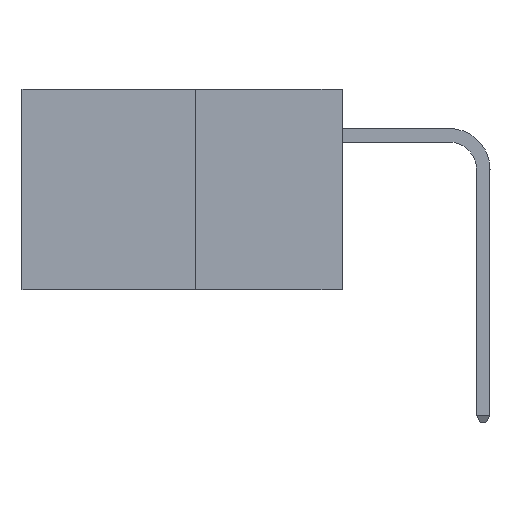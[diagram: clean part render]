
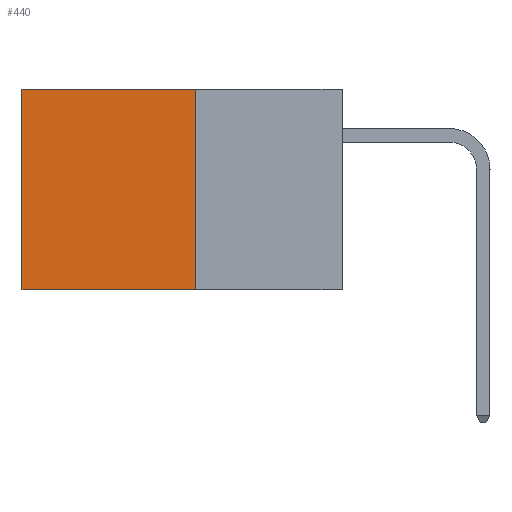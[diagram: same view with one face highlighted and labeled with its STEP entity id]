
A CAD part, left-side view. The second image highlights one B-rep face of the part: STEP entity #440.
In plain terms, the highlighted planar face has unit normal (-1, 0, 0).
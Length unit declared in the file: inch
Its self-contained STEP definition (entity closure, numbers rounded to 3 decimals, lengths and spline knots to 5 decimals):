
#440 = ADVANCED_FACE ( 'NONE', ( #1558 ), #6231, .F. ) ;
#591 = VERTEX_POINT ( 'NONE', #8711 ) ;
#705 = CARTESIAN_POINT ( 'NONE',  ( 0.277, 0.59, -0.37 ) ) ;
#973 = LINE ( 'NONE', #4174, #2539 ) ;
#1151 = AXIS2_PLACEMENT_3D ( 'NONE', #6105, #7472, #7715 ) ;
#1262 = VECTOR ( 'NONE', #6372, 39.37008 ) ;
#1380 = EDGE_CURVE ( 'NONE', #5025, #4169, #5821, .T. ) ;
#1461 = EDGE_CURVE ( 'NONE', #591, #5025, #973, .T. ) ;
#1558 = FACE_OUTER_BOUND ( 'NONE', #2930, .T. ) ;
#2422 = CARTESIAN_POINT ( 'NONE',  ( 0.277, 0.59, 0. ) ) ;
#2539 = VECTOR ( 'NONE', #3127, 39.37008 ) ;
#2930 = EDGE_LOOP ( 'NONE', ( #3466, #8138, #5736, #7564 ) ) ;
#3030 = EDGE_CURVE ( 'NONE', #591, #8297, #7572, .T. ) ;
#3127 = DIRECTION ( 'NONE',  ( 0., 1., 0. ) ) ;
#3139 = CARTESIAN_POINT ( 'NONE',  ( 0.277, 0.27, -0.37 ) ) ;
#3466 = ORIENTED_EDGE ( 'NONE', *, *, #1380, .T. ) ;
#4165 = DIRECTION ( 'NONE',  ( 0., 1., 0. ) ) ;
#4169 = VERTEX_POINT ( 'NONE', #705 ) ;
#4174 = CARTESIAN_POINT ( 'NONE',  ( 0.277, 0.27, 0. ) ) ;
#4179 = VECTOR ( 'NONE', #4165, 39.37008 ) ;
#5025 = VERTEX_POINT ( 'NONE', #2422 ) ;
#5084 = EDGE_CURVE ( 'NONE', #8297, #4169, #8016, .T. ) ;
#5736 = ORIENTED_EDGE ( 'NONE', *, *, #3030, .F. ) ;
#5821 = LINE ( 'NONE', #6593, #1262 ) ;
#5828 = VECTOR ( 'NONE', #8293, 39.37008 ) ;
#6105 = CARTESIAN_POINT ( 'NONE',  ( 0.277, 0.27, -0.37 ) ) ;
#6231 = PLANE ( 'NONE',  #1151 ) ;
#6372 = DIRECTION ( 'NONE',  ( 0., 0., -1. ) ) ;
#6593 = CARTESIAN_POINT ( 'NONE',  ( 0.277, 0.59, -0.37 ) ) ;
#7472 = DIRECTION ( 'NONE',  ( 1., 0., 0. ) ) ;
#7564 = ORIENTED_EDGE ( 'NONE', *, *, #1461, .T. ) ;
#7572 = LINE ( 'NONE', #8471, #5828 ) ;
#7604 = CARTESIAN_POINT ( 'NONE',  ( 0.277, 0.27, -0.37 ) ) ;
#7715 = DIRECTION ( 'NONE',  ( 0., 0., -1. ) ) ;
#8016 = LINE ( 'NONE', #7604, #4179 ) ;
#8138 = ORIENTED_EDGE ( 'NONE', *, *, #5084, .F. ) ;
#8293 = DIRECTION ( 'NONE',  ( 0., 0., -1. ) ) ;
#8297 = VERTEX_POINT ( 'NONE', #3139 ) ;
#8471 = CARTESIAN_POINT ( 'NONE',  ( 0.277, 0.27, -0.37 ) ) ;
#8711 = CARTESIAN_POINT ( 'NONE',  ( 0.277, 0.27, 0. ) ) ;
